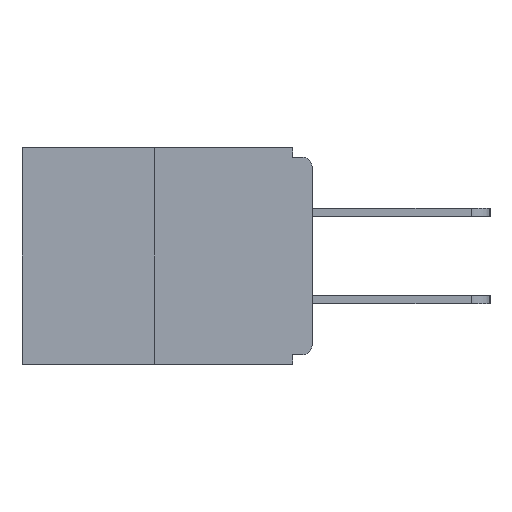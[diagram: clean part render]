
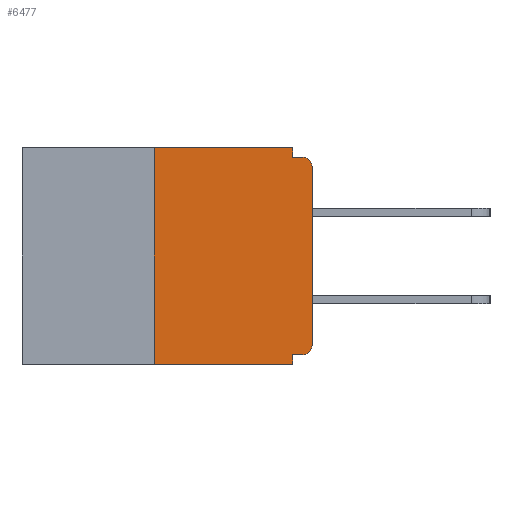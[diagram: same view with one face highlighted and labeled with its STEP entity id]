
A CAD part, left-side view. The second image highlights one B-rep face of the part: STEP entity #6477.
In plain terms, the highlighted planar face has unit normal (-1, 0, 0).
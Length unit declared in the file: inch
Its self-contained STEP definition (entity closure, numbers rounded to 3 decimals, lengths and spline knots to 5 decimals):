
#470 = VERTEX_POINT ( 'NONE', #13379 ) ;
#544 = DIRECTION ( 'NONE',  ( 0., -1., 0. ) ) ;
#613 = LINE ( 'NONE', #14530, #4408 ) ;
#762 = DIRECTION ( 'NONE',  ( -1., 0., 0. ) ) ;
#802 = ORIENTED_EDGE ( 'NONE', *, *, #10180, .F. ) ;
#1053 = ORIENTED_EDGE ( 'NONE', *, *, #3858, .T. ) ;
#1215 = VECTOR ( 'NONE', #7270, 39.37008 ) ;
#1247 = CARTESIAN_POINT ( 'NONE',  ( 0., 0.015, -0.015 ) ) ;
#1258 = LINE ( 'NONE', #15177, #1215 ) ;
#1332 = AXIS2_PLACEMENT_3D ( 'NONE', #12447, #762, #6637 ) ;
#2452 = DIRECTION ( 'NONE',  ( 0., -1., 0. ) ) ;
#2627 = CARTESIAN_POINT ( 'NONE',  ( 0., 0.46, -0.343 ) ) ;
#2710 = CARTESIAN_POINT ( 'NONE',  ( 0., 0.015, -0.328 ) ) ;
#2961 = VECTOR ( 'NONE', #6268, 39.37008 ) ;
#3182 = PLANE ( 'NONE',  #13085 ) ;
#3208 = ORIENTED_EDGE ( 'NONE', *, *, #7533, .F. ) ;
#3364 = ORIENTED_EDGE ( 'NONE', *, *, #13890, .F. ) ;
#3458 = VERTEX_POINT ( 'NONE', #7699 ) ;
#3747 = EDGE_CURVE ( 'NONE', #5607, #11964, #4938, .T. ) ;
#3811 = VECTOR ( 'NONE', #7604, 39.37008 ) ;
#3858 = EDGE_CURVE ( 'NONE', #10293, #8204, #10190, .T. ) ;
#4002 = CARTESIAN_POINT ( 'NONE',  ( 0., 0., -0.328 ) ) ;
#4008 = DIRECTION ( 'NONE',  ( 0., 0., -1. ) ) ;
#4192 = CARTESIAN_POINT ( 'NONE',  ( 0., 0.46, 0. ) ) ;
#4408 = VECTOR ( 'NONE', #4008, 39.37008 ) ;
#4549 = EDGE_CURVE ( 'NONE', #470, #10618, #9640, .T. ) ;
#4938 = LINE ( 'NONE', #13061, #8766 ) ;
#5068 = CIRCLE ( 'NONE', #13630, 0.015 ) ;
#5087 = VECTOR ( 'NONE', #5426, 39.37008 ) ;
#5292 = VERTEX_POINT ( 'NONE', #8180 ) ;
#5303 = CARTESIAN_POINT ( 'NONE',  ( 0., 0., -0.015 ) ) ;
#5426 = DIRECTION ( 'NONE',  ( 0., 0., 1. ) ) ;
#5581 = DIRECTION ( 'NONE',  ( 1., 0., 0. ) ) ;
#5607 = VERTEX_POINT ( 'NONE', #14838 ) ;
#5815 = ORIENTED_EDGE ( 'NONE', *, *, #4549, .F. ) ;
#6068 = CARTESIAN_POINT ( 'NONE',  ( 0., 0.031, 0. ) ) ;
#6141 = EDGE_CURVE ( 'NONE', #3458, #5607, #1258, .T. ) ;
#6163 = ORIENTED_EDGE ( 'NONE', *, *, #6644, .T. ) ;
#6268 = DIRECTION ( 'NONE',  ( 0., 0., -1. ) ) ;
#6477 = ADVANCED_FACE ( 'NONE', ( #13699 ), #3182, .F. ) ;
#6637 = DIRECTION ( 'NONE',  ( 0., 0., -1. ) ) ;
#6644 = EDGE_CURVE ( 'NONE', #11256, #5292, #5068, .T. ) ;
#6708 = EDGE_CURVE ( 'NONE', #3458, #10618, #14462, .T. ) ;
#6765 = VERTEX_POINT ( 'NONE', #13234 ) ;
#6797 = VECTOR ( 'NONE', #544, 39.37008 ) ;
#7248 = CARTESIAN_POINT ( 'NONE',  ( 0., 0.031, -0.343 ) ) ;
#7250 = ORIENTED_EDGE ( 'NONE', *, *, #6141, .F. ) ;
#7270 = DIRECTION ( 'NONE',  ( 0., 0., 1. ) ) ;
#7533 = EDGE_CURVE ( 'NONE', #11256, #470, #10926, .T. ) ;
#7604 = DIRECTION ( 'NONE',  ( 0., -1., 0. ) ) ;
#7699 = CARTESIAN_POINT ( 'NONE',  ( 0., 0.25, -0.343 ) ) ;
#7784 = VECTOR ( 'NONE', #14447, 39.37008 ) ;
#7876 = DIRECTION ( 'NONE',  ( 0., 0., -1. ) ) ;
#7931 = CARTESIAN_POINT ( 'NONE',  ( 0., 0., 0. ) ) ;
#8108 = CARTESIAN_POINT ( 'NONE',  ( 0., 0.015, -0.313 ) ) ;
#8180 = CARTESIAN_POINT ( 'NONE',  ( 0., 0., -0.313 ) ) ;
#8204 = VERTEX_POINT ( 'NONE', #1247 ) ;
#8232 = ORIENTED_EDGE ( 'NONE', *, *, #6708, .T. ) ;
#8509 = ORIENTED_EDGE ( 'NONE', *, *, #11403, .T. ) ;
#8766 = VECTOR ( 'NONE', #2452, 39.37008 ) ;
#8915 = LINE ( 'NONE', #5303, #3811 ) ;
#9295 = ORIENTED_EDGE ( 'NONE', *, *, #3747, .F. ) ;
#9640 = LINE ( 'NONE', #7248, #2961 ) ;
#9817 = CARTESIAN_POINT ( 'NONE',  ( 0., 0.031, -0.343 ) ) ;
#10180 = EDGE_CURVE ( 'NONE', #6765, #8204, #8915, .T. ) ;
#10190 = CIRCLE ( 'NONE', #1332, 0.015 ) ;
#10293 = VERTEX_POINT ( 'NONE', #14033 ) ;
#10618 = VERTEX_POINT ( 'NONE', #9817 ) ;
#10635 = DIRECTION ( 'NONE',  ( -1., 0., 0. ) ) ;
#10926 = LINE ( 'NONE', #4002, #7784 ) ;
#11256 = VERTEX_POINT ( 'NONE', #2710 ) ;
#11403 = EDGE_CURVE ( 'NONE', #5292, #10293, #13760, .T. ) ;
#11964 = VERTEX_POINT ( 'NONE', #6068 ) ;
#12447 = CARTESIAN_POINT ( 'NONE',  ( 0., 0.015, -0.03 ) ) ;
#12783 = DIRECTION ( 'NONE',  ( 0., 0., -1. ) ) ;
#13061 = CARTESIAN_POINT ( 'NONE',  ( 0., 0.46, 0. ) ) ;
#13085 = AXIS2_PLACEMENT_3D ( 'NONE', #4192, #5581, #7876 ) ;
#13234 = CARTESIAN_POINT ( 'NONE',  ( 0., 0.031, -0.015 ) ) ;
#13379 = CARTESIAN_POINT ( 'NONE',  ( 0., 0.031, -0.328 ) ) ;
#13418 = EDGE_LOOP ( 'NONE', ( #9295, #7250, #8232, #5815, #3208, #6163, #8509, #1053, #802, #3364 ) ) ;
#13630 = AXIS2_PLACEMENT_3D ( 'NONE', #8108, #10635, #12783 ) ;
#13699 = FACE_OUTER_BOUND ( 'NONE', #13418, .T. ) ;
#13760 = LINE ( 'NONE', #7931, #5087 ) ;
#13890 = EDGE_CURVE ( 'NONE', #11964, #6765, #613, .T. ) ;
#14033 = CARTESIAN_POINT ( 'NONE',  ( 0., 0., -0.03 ) ) ;
#14447 = DIRECTION ( 'NONE',  ( 0., 1., 0. ) ) ;
#14462 = LINE ( 'NONE', #2627, #6797 ) ;
#14530 = CARTESIAN_POINT ( 'NONE',  ( 0., 0.031, 0. ) ) ;
#14838 = CARTESIAN_POINT ( 'NONE',  ( 0., 0.25, 0. ) ) ;
#15177 = CARTESIAN_POINT ( 'NONE',  ( 0., 0.25, 0. ) ) ;
